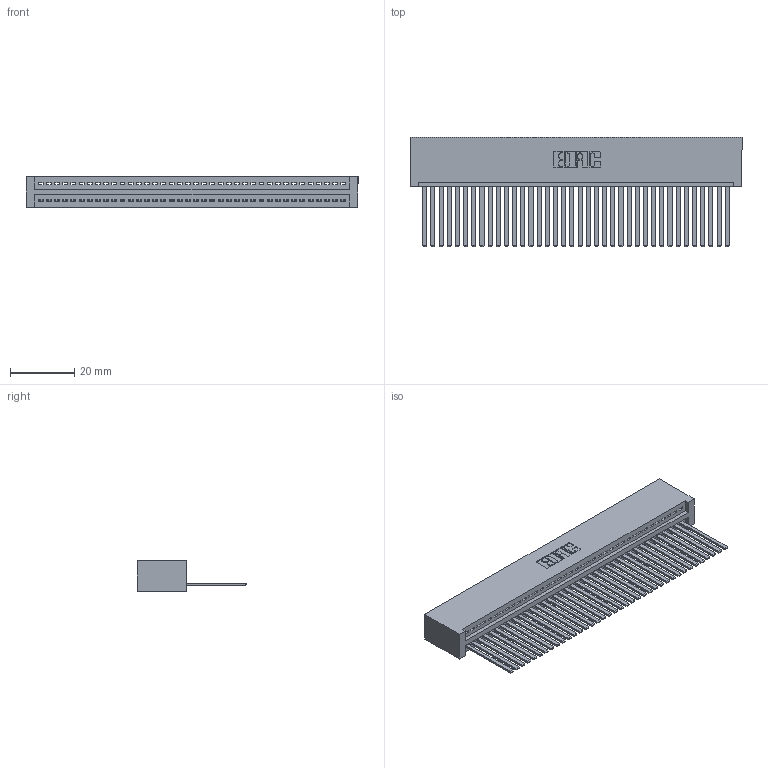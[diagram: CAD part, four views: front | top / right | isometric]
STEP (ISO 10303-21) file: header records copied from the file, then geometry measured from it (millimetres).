
FILE_DESCRIPTION (( 'STEP AP203' ), '1' );
FILE_NAME ('345-038-544-101.STEP', '2018-08-30T08:40:32', ( '' ), ( '' ), 'SwSTEP 2.0', 'SolidWorks 2016', '' );
FILE_SCHEMA (( 'CONFIG_CONTROL_DESIGN' ));
Length unit declared in the file: inch
Products named in the file (3): 345 Part_No Mounting Lugs; 345-292-001_345-293-144; 345-038-544-101
Assembly tree (39 placements, depth 2):
  345-038-544-101
    345 Part_No Mounting Lugs
    345-292-001_345-293-144  x38
Bounding box: 103.12 x 33.96 x 9.4 mm (x, y, z)
Volume: 10786.5 mm3; surface area: 15791.3 mm2
Topology: 39 solids, 39 shells, 2094 faces, 6321 edges, 4162 vertices
Faces by surface type: plane 1444, cylinder 650
Entity records: 28677 total; most frequent: CARTESIAN_POINT 4974, ORIENTED_EDGE 4946, DIRECTION 4341, EDGE_CURVE 2473, LINE 2201, VECTOR 2201, VERTEX_POINT 1646, AXIS2_PLACEMENT_3D 1070
